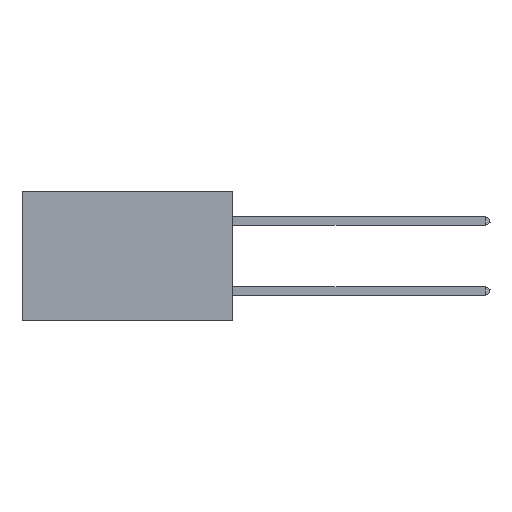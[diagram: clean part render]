
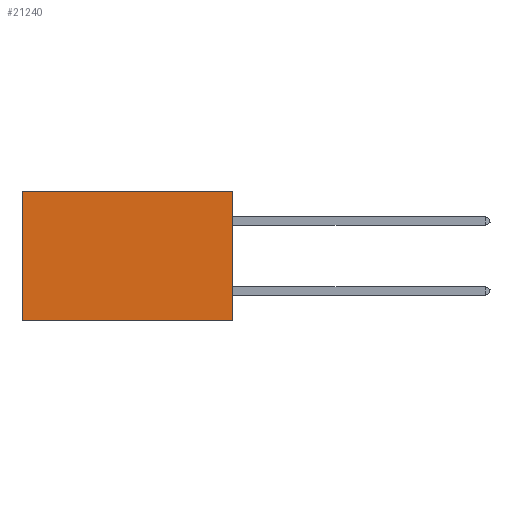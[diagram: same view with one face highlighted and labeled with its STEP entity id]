
A CAD part, left-side view. The second image highlights one B-rep face of the part: STEP entity #21240.
In plain terms, the highlighted planar face has unit normal (-1, 0, 0).
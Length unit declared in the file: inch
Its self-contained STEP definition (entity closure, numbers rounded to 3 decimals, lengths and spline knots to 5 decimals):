
#432 = EDGE_CURVE ( 'NONE', #37639, #14849, #36520, .T. ) ;
#1476 = LINE ( 'NONE', #22134, #37174 ) ;
#2047 = FACE_OUTER_BOUND ( 'NONE', #3261, .T. ) ;
#3261 = EDGE_LOOP ( 'NONE', ( #17206, #34021, #3674, #16764 ) ) ;
#3674 = ORIENTED_EDGE ( 'NONE', *, *, #12984, .F. ) ;
#3789 = VECTOR ( 'NONE', #22752, 39.37008 ) ;
#5538 = DIRECTION ( 'NONE',  ( 1., 0., 0. ) ) ;
#5642 = LINE ( 'NONE', #11208, #3789 ) ;
#6268 = VERTEX_POINT ( 'NONE', #30213 ) ;
#7348 = VECTOR ( 'NONE', #34907, 39.37008 ) ;
#8802 = LINE ( 'NONE', #25931, #24054 ) ;
#11040 = CARTESIAN_POINT ( 'NONE',  ( 0.2875, 0., -0.37 ) ) ;
#11208 = CARTESIAN_POINT ( 'NONE',  ( 0.2875, 0.6, 0. ) ) ;
#11798 = EDGE_CURVE ( 'NONE', #21601, #14849, #5642, .T. ) ;
#12984 = EDGE_CURVE ( 'NONE', #6268, #37639, #8802, .T. ) ;
#14849 = VERTEX_POINT ( 'NONE', #16442 ) ;
#16442 = CARTESIAN_POINT ( 'NONE',  ( 0.2875, 0.6, -0.37 ) ) ;
#16764 = ORIENTED_EDGE ( 'NONE', *, *, #34799, .T. ) ;
#16846 = DIRECTION ( 'NONE',  ( 0., 0., -1. ) ) ;
#17181 = CARTESIAN_POINT ( 'NONE',  ( 0.2875, 0., 0. ) ) ;
#17206 = ORIENTED_EDGE ( 'NONE', *, *, #11798, .T. ) ;
#21240 = ADVANCED_FACE ( 'NONE', ( #2047 ), #26155, .F. ) ;
#21601 = VERTEX_POINT ( 'NONE', #22074 ) ;
#22074 = CARTESIAN_POINT ( 'NONE',  ( 0.2875, 0.6, 0. ) ) ;
#22134 = CARTESIAN_POINT ( 'NONE',  ( 0.2875, 0., 0. ) ) ;
#22752 = DIRECTION ( 'NONE',  ( 0., 0., -1. ) ) ;
#24054 = VECTOR ( 'NONE', #16846, 39.37008 ) ;
#24123 = CARTESIAN_POINT ( 'NONE',  ( 0.2875, 0., -0.37 ) ) ;
#25931 = CARTESIAN_POINT ( 'NONE',  ( 0.2875, 0., 0. ) ) ;
#26155 = PLANE ( 'NONE',  #37388 ) ;
#26288 = DIRECTION ( 'NONE',  ( 0., 0., -1. ) ) ;
#30213 = CARTESIAN_POINT ( 'NONE',  ( 0.2875, 0., 0. ) ) ;
#31084 = DIRECTION ( 'NONE',  ( 0., 1., 0. ) ) ;
#34021 = ORIENTED_EDGE ( 'NONE', *, *, #432, .F. ) ;
#34799 = EDGE_CURVE ( 'NONE', #6268, #21601, #1476, .T. ) ;
#34907 = DIRECTION ( 'NONE',  ( 0., 1., 0. ) ) ;
#36520 = LINE ( 'NONE', #11040, #7348 ) ;
#37174 = VECTOR ( 'NONE', #31084, 39.37008 ) ;
#37388 = AXIS2_PLACEMENT_3D ( 'NONE', #17181, #5538, #26288 ) ;
#37639 = VERTEX_POINT ( 'NONE', #24123 ) ;
